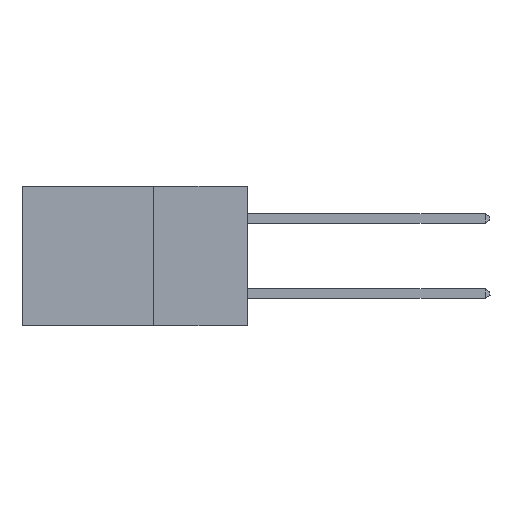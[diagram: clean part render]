
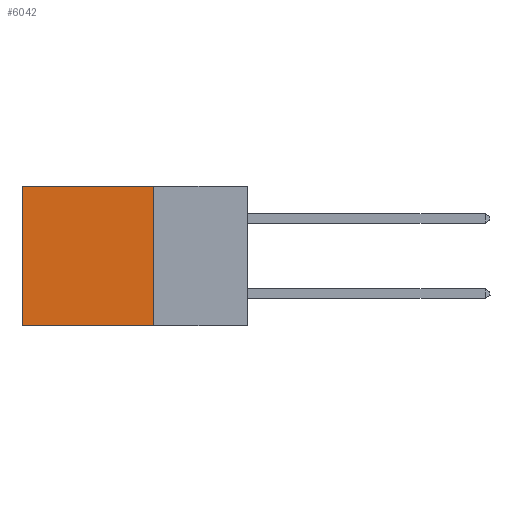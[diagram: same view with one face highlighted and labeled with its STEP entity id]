
A CAD part, left-side view. The second image highlights one B-rep face of the part: STEP entity #6042.
In plain terms, the highlighted planar face has unit normal (-1, 0, 0).
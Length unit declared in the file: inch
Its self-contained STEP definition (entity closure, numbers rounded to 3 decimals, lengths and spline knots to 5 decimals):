
#459 = ORIENTED_EDGE ( 'NONE', *, *, #7578, .F. ) ;
#1583 = LINE ( 'NONE', #10736, #8102 ) ;
#1986 = VERTEX_POINT ( 'NONE', #6870 ) ;
#2017 = CARTESIAN_POINT ( 'NONE',  ( 0.298, 0.25, -0.37 ) ) ;
#2223 = VERTEX_POINT ( 'NONE', #5939 ) ;
#2514 = ORIENTED_EDGE ( 'NONE', *, *, #11461, .F. ) ;
#2539 = EDGE_CURVE ( 'NONE', #10091, #2223, #5782, .T. ) ;
#2804 = LINE ( 'NONE', #6032, #12248 ) ;
#2957 = DIRECTION ( 'NONE',  ( 0., 1., 0. ) ) ;
#3117 = DIRECTION ( 'NONE',  ( 0., 0., -1. ) ) ;
#3447 = EDGE_LOOP ( 'NONE', ( #5595, #459, #2514, #5377 ) ) ;
#3452 = CARTESIAN_POINT ( 'NONE',  ( 0.298, 0.25, 0. ) ) ;
#3493 = VERTEX_POINT ( 'NONE', #2017 ) ;
#4185 = PLANE ( 'NONE',  #11691 ) ;
#4999 = VECTOR ( 'NONE', #10743, 39.37008 ) ;
#5377 = ORIENTED_EDGE ( 'NONE', *, *, #2539, .T. ) ;
#5595 = ORIENTED_EDGE ( 'NONE', *, *, #8039, .T. ) ;
#5657 = LINE ( 'NONE', #8683, #10647 ) ;
#5782 = LINE ( 'NONE', #9662, #4999 ) ;
#5939 = CARTESIAN_POINT ( 'NONE',  ( 0.298, 0.6, 0. ) ) ;
#6029 = DIRECTION ( 'NONE',  ( 1., 0., 0. ) ) ;
#6032 = CARTESIAN_POINT ( 'NONE',  ( 0.298, 0.25, -0.37 ) ) ;
#6042 = ADVANCED_FACE ( 'NONE', ( #12773 ), #4185, .F. ) ;
#6870 = CARTESIAN_POINT ( 'NONE',  ( 0.298, 0.6, -0.37 ) ) ;
#7578 = EDGE_CURVE ( 'NONE', #3493, #1986, #2804, .T. ) ;
#8039 = EDGE_CURVE ( 'NONE', #2223, #1986, #5657, .T. ) ;
#8099 = DIRECTION ( 'NONE',  ( 0., 0., -1. ) ) ;
#8102 = VECTOR ( 'NONE', #3117, 39.37008 ) ;
#8683 = CARTESIAN_POINT ( 'NONE',  ( 0.298, 0.6, 0. ) ) ;
#9662 = CARTESIAN_POINT ( 'NONE',  ( 0.298, 0.25, 0. ) ) ;
#10091 = VERTEX_POINT ( 'NONE', #3452 ) ;
#10187 = CARTESIAN_POINT ( 'NONE',  ( 0.298, 0.25, 0. ) ) ;
#10647 = VECTOR ( 'NONE', #11768, 39.37008 ) ;
#10736 = CARTESIAN_POINT ( 'NONE',  ( 0.298, 0.25, 0. ) ) ;
#10743 = DIRECTION ( 'NONE',  ( 0., 1., 0. ) ) ;
#11461 = EDGE_CURVE ( 'NONE', #10091, #3493, #1583, .T. ) ;
#11691 = AXIS2_PLACEMENT_3D ( 'NONE', #10187, #6029, #8099 ) ;
#11768 = DIRECTION ( 'NONE',  ( 0., 0., -1. ) ) ;
#12248 = VECTOR ( 'NONE', #2957, 39.37008 ) ;
#12773 = FACE_OUTER_BOUND ( 'NONE', #3447, .T. ) ;
